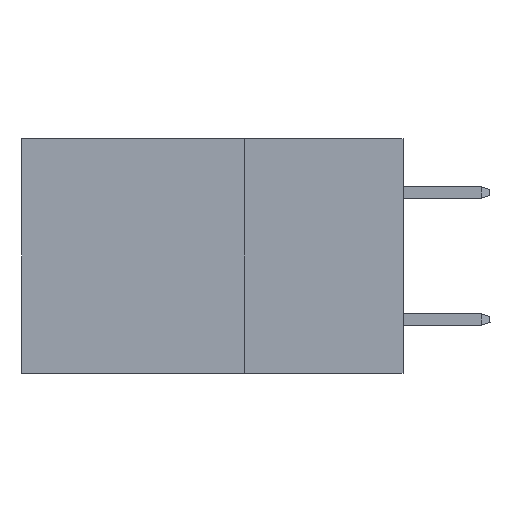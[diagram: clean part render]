
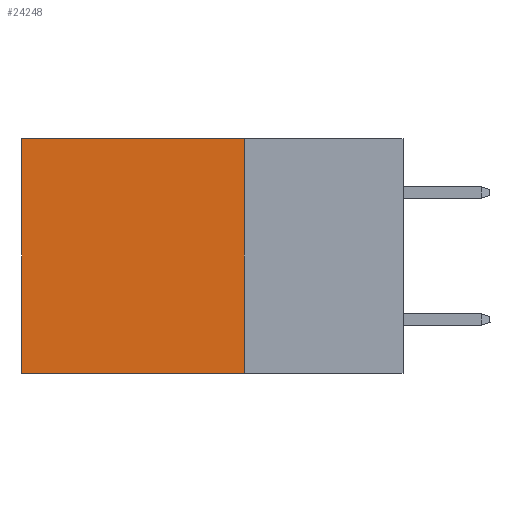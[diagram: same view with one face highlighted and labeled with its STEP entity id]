
A CAD part, left-side view. The second image highlights one B-rep face of the part: STEP entity #24248.
In plain terms, the highlighted planar face has unit normal (-1, 0, 0).
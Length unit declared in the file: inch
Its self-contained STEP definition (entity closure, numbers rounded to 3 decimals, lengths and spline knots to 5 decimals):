
#1337 = LINE ( 'NONE', #5492, #26484 ) ;
#2692 = EDGE_CURVE ( 'NONE', #26211, #5417, #13297, .T. ) ;
#4604 = EDGE_CURVE ( 'NONE', #8572, #26211, #16484, .T. ) ;
#5417 = VERTEX_POINT ( 'NONE', #9474 ) ;
#5492 = CARTESIAN_POINT ( 'NONE',  ( 0.2875, 0.25, 0. ) ) ;
#5763 = DIRECTION ( 'NONE',  ( 0., 1., 0. ) ) ;
#6785 = EDGE_CURVE ( 'NONE', #18920, #5417, #13634, .T. ) ;
#6851 = DIRECTION ( 'NONE',  ( 0., 0., -1. ) ) ;
#7537 = VECTOR ( 'NONE', #13243, 39.37008 ) ;
#8195 = DIRECTION ( 'NONE',  ( 0., 0., -1. ) ) ;
#8572 = VERTEX_POINT ( 'NONE', #20936 ) ;
#8881 = DIRECTION ( 'NONE',  ( 0., 1., 0. ) ) ;
#9474 = CARTESIAN_POINT ( 'NONE',  ( 0.2875, 0.6, -0.37 ) ) ;
#9832 = CARTESIAN_POINT ( 'NONE',  ( 0.2875, 0.25, 0. ) ) ;
#10718 = DIRECTION ( 'NONE',  ( 1., 0., 0. ) ) ;
#12266 = ORIENTED_EDGE ( 'NONE', *, *, #2692, .F. ) ;
#12592 = PLANE ( 'NONE',  #18263 ) ;
#12991 = CARTESIAN_POINT ( 'NONE',  ( 0.2875, 0.25, 0. ) ) ;
#13243 = DIRECTION ( 'NONE',  ( 0., 0., -1. ) ) ;
#13297 = LINE ( 'NONE', #25276, #13386 ) ;
#13386 = VECTOR ( 'NONE', #8881, 39.37008 ) ;
#13634 = LINE ( 'NONE', #15658, #7537 ) ;
#15658 = CARTESIAN_POINT ( 'NONE',  ( 0.2875, 0.6, 0. ) ) ;
#16462 = EDGE_CURVE ( 'NONE', #8572, #18920, #1337, .T. ) ;
#16484 = LINE ( 'NONE', #9832, #21213 ) ;
#17393 = CARTESIAN_POINT ( 'NONE',  ( 0.2875, 0.25, -0.37 ) ) ;
#17719 = ORIENTED_EDGE ( 'NONE', *, *, #16462, .T. ) ;
#18263 = AXIS2_PLACEMENT_3D ( 'NONE', #12991, #10718, #6851 ) ;
#18880 = EDGE_LOOP ( 'NONE', ( #19419, #12266, #21158, #17719 ) ) ;
#18920 = VERTEX_POINT ( 'NONE', #20876 ) ;
#19419 = ORIENTED_EDGE ( 'NONE', *, *, #6785, .T. ) ;
#20876 = CARTESIAN_POINT ( 'NONE',  ( 0.2875, 0.6, 0. ) ) ;
#20936 = CARTESIAN_POINT ( 'NONE',  ( 0.2875, 0.25, 0. ) ) ;
#21158 = ORIENTED_EDGE ( 'NONE', *, *, #4604, .F. ) ;
#21213 = VECTOR ( 'NONE', #8195, 39.37008 ) ;
#24248 = ADVANCED_FACE ( 'NONE', ( #24962 ), #12592, .F. ) ;
#24962 = FACE_OUTER_BOUND ( 'NONE', #18880, .T. ) ;
#25276 = CARTESIAN_POINT ( 'NONE',  ( 0.2875, 0.25, -0.37 ) ) ;
#26211 = VERTEX_POINT ( 'NONE', #17393 ) ;
#26484 = VECTOR ( 'NONE', #5763, 39.37008 ) ;
